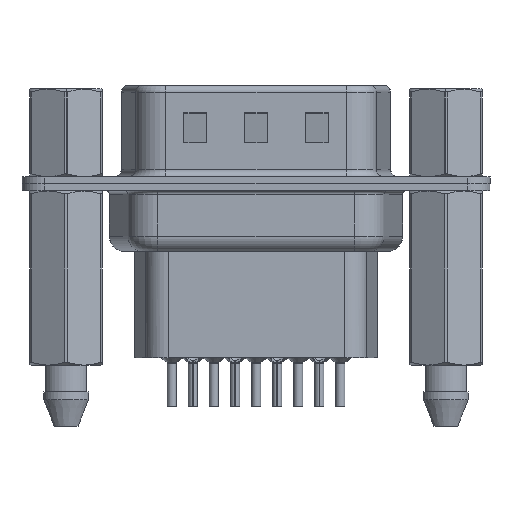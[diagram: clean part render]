
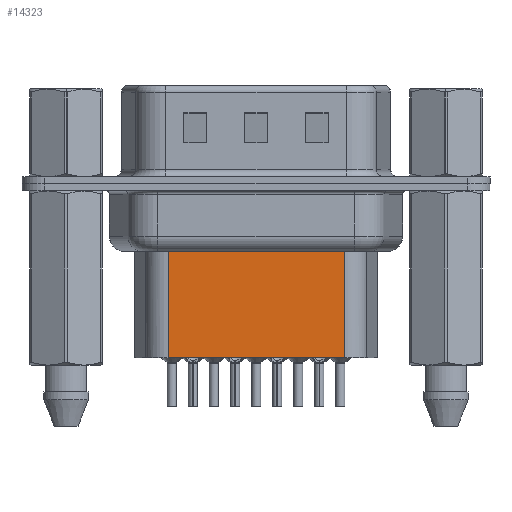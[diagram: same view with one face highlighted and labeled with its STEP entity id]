
A CAD part, front view. The second image highlights one B-rep face of the part: STEP entity #14323.
In plain terms, the highlighted planar face has unit normal (0, -1, 0).
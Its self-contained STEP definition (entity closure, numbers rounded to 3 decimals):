
#185 = PLANE ( 'NONE',  #25847 ) ;
#306 = CARTESIAN_POINT ( 'NONE',  ( 6.459, -3.5, -4.097 ) ) ;
#1301 = DIRECTION ( 'NONE',  ( -1., 0., 0. ) ) ;
#1706 = EDGE_CURVE ( 'NONE', #8862, #9090, #17158, .T. ) ;
#2237 = DIRECTION ( 'NONE',  ( 1., 0., 0. ) ) ;
#2283 = VERTEX_POINT ( 'NONE', #6077 ) ;
#3542 = ORIENTED_EDGE ( 'NONE', *, *, #16053, .T. ) ;
#3705 = CARTESIAN_POINT ( 'NONE',  ( 18.294, -3.5, -11.45 ) ) ;
#4239 = LINE ( 'NONE', #306, #19641 ) ;
#6077 = CARTESIAN_POINT ( 'NONE',  ( 6.706, -3.5, -4.097 ) ) ;
#6208 = CARTESIAN_POINT ( 'NONE',  ( 6.706, -3.5, -3.1 ) ) ;
#6529 = VERTEX_POINT ( 'NONE', #19135 ) ;
#6946 = EDGE_CURVE ( 'NONE', #6529, #2283, #4239, .T. ) ;
#8238 = DIRECTION ( 'NONE',  ( 0., 0., -1. ) ) ;
#8376 = LINE ( 'NONE', #6208, #18415 ) ;
#8862 = VERTEX_POINT ( 'NONE', #3705 ) ;
#9090 = VERTEX_POINT ( 'NONE', #13290 ) ;
#10021 = FACE_OUTER_BOUND ( 'NONE', #23326, .T. ) ;
#10224 = CARTESIAN_POINT ( 'NONE',  ( 6.706, -3.5, -3.1 ) ) ;
#13290 = CARTESIAN_POINT ( 'NONE',  ( 6.706, -3.5, -11.45 ) ) ;
#13597 = CARTESIAN_POINT ( 'NONE',  ( 18.294, -3.5, -3.1 ) ) ;
#13646 = EDGE_CURVE ( 'NONE', #6529, #8862, #26088, .T. ) ;
#14134 = DIRECTION ( 'NONE',  ( 0., 0., -1. ) ) ;
#14273 = DIRECTION ( 'NONE',  ( 0., -1., 0. ) ) ;
#14323 = ADVANCED_FACE ( 'NONE', ( #10021 ), #185, .T. ) ;
#15669 = ORIENTED_EDGE ( 'NONE', *, *, #13646, .F. ) ;
#16053 = EDGE_CURVE ( 'NONE', #2283, #9090, #8376, .T. ) ;
#16555 = VECTOR ( 'NONE', #1301, 1000. ) ;
#17158 = LINE ( 'NONE', #23106, #16555 ) ;
#18415 = VECTOR ( 'NONE', #8238, 1000. ) ;
#19135 = CARTESIAN_POINT ( 'NONE',  ( 18.294, -3.5, -4.097 ) ) ;
#19452 = ORIENTED_EDGE ( 'NONE', *, *, #6946, .T. ) ;
#19641 = VECTOR ( 'NONE', #22404, 1000. ) ;
#20723 = VECTOR ( 'NONE', #14134, 1000. ) ;
#20816 = ORIENTED_EDGE ( 'NONE', *, *, #1706, .F. ) ;
#22404 = DIRECTION ( 'NONE',  ( -1., 0., 0. ) ) ;
#23106 = CARTESIAN_POINT ( 'NONE',  ( 6.706, -3.5, -11.45 ) ) ;
#23326 = EDGE_LOOP ( 'NONE', ( #15669, #19452, #3542, #20816 ) ) ;
#25847 = AXIS2_PLACEMENT_3D ( 'NONE', #10224, #14273, #2237 ) ;
#26088 = LINE ( 'NONE', #13597, #20723 ) ;
